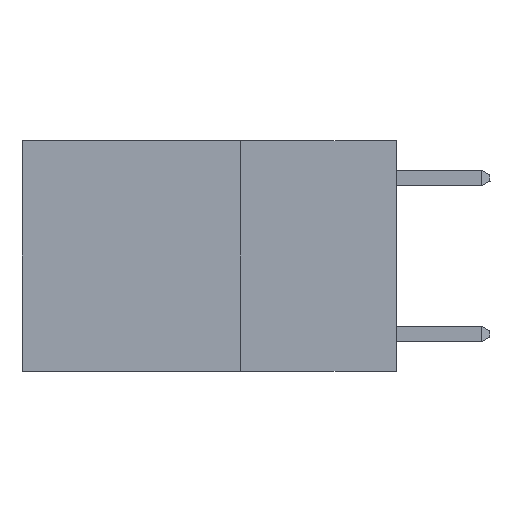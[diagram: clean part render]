
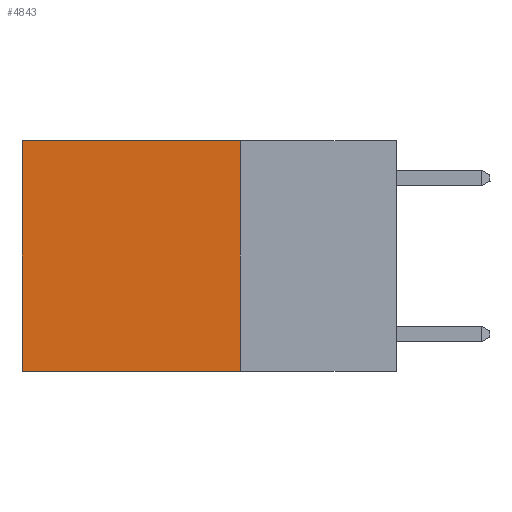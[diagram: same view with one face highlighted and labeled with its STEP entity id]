
A CAD part, left-side view. The second image highlights one B-rep face of the part: STEP entity #4843.
In plain terms, the highlighted planar face has unit normal (-1, 0, 0).
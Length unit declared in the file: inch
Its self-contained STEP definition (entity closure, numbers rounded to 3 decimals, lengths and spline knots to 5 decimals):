
#324 = EDGE_LOOP ( 'NONE', ( #731, #6170, #7046, #10749 ) ) ;
#694 = CARTESIAN_POINT ( 'NONE',  ( 0.2625, 0.25, 0. ) ) ;
#731 = ORIENTED_EDGE ( 'NONE', *, *, #8200, .T. ) ;
#761 = CARTESIAN_POINT ( 'NONE',  ( 0.2625, 0.25, 0. ) ) ;
#950 = DIRECTION ( 'NONE',  ( 0., 1., 0. ) ) ;
#1042 = LINE ( 'NONE', #694, #6366 ) ;
#1320 = DIRECTION ( 'NONE',  ( 0., 0., -1. ) ) ;
#1477 = CARTESIAN_POINT ( 'NONE',  ( 0.2625, 0.6, 0. ) ) ;
#1602 = CARTESIAN_POINT ( 'NONE',  ( 0.2625, 0.25, 0. ) ) ;
#2313 = DIRECTION ( 'NONE',  ( 0., 0., -1. ) ) ;
#2990 = AXIS2_PLACEMENT_3D ( 'NONE', #761, #7392, #2313 ) ;
#3279 = CARTESIAN_POINT ( 'NONE',  ( 0.2625, 0.25, -0.37 ) ) ;
#3387 = LINE ( 'NONE', #4454, #7149 ) ;
#3473 = LINE ( 'NONE', #10647, #9491 ) ;
#3931 = EDGE_CURVE ( 'NONE', #10373, #10743, #11001, .T. ) ;
#4454 = CARTESIAN_POINT ( 'NONE',  ( 0.2625, 0.25, 0. ) ) ;
#4843 = ADVANCED_FACE ( 'NONE', ( #4949 ), #4900, .F. ) ;
#4900 = PLANE ( 'NONE',  #2990 ) ;
#4949 = FACE_OUTER_BOUND ( 'NONE', #324, .T. ) ;
#6170 = ORIENTED_EDGE ( 'NONE', *, *, #3931, .F. ) ;
#6366 = VECTOR ( 'NONE', #10824, 39.37008 ) ;
#6766 = EDGE_CURVE ( 'NONE', #7752, #9865, #3387, .T. ) ;
#7046 = ORIENTED_EDGE ( 'NONE', *, *, #7432, .F. ) ;
#7149 = VECTOR ( 'NONE', #10443, 39.37008 ) ;
#7392 = DIRECTION ( 'NONE',  ( 1., 0., 0. ) ) ;
#7432 = EDGE_CURVE ( 'NONE', #7752, #10373, #1042, .T. ) ;
#7488 = CARTESIAN_POINT ( 'NONE',  ( 0.2625, 0.6, -0.37 ) ) ;
#7752 = VERTEX_POINT ( 'NONE', #1602 ) ;
#8200 = EDGE_CURVE ( 'NONE', #9865, #10743, #3473, .T. ) ;
#9491 = VECTOR ( 'NONE', #1320, 39.37008 ) ;
#9865 = VERTEX_POINT ( 'NONE', #1477 ) ;
#10373 = VERTEX_POINT ( 'NONE', #10933 ) ;
#10443 = DIRECTION ( 'NONE',  ( 0., 1., 0. ) ) ;
#10647 = CARTESIAN_POINT ( 'NONE',  ( 0.2625, 0.6, 0. ) ) ;
#10731 = VECTOR ( 'NONE', #950, 39.37008 ) ;
#10743 = VERTEX_POINT ( 'NONE', #7488 ) ;
#10749 = ORIENTED_EDGE ( 'NONE', *, *, #6766, .T. ) ;
#10824 = DIRECTION ( 'NONE',  ( 0., 0., -1. ) ) ;
#10933 = CARTESIAN_POINT ( 'NONE',  ( 0.2625, 0.25, -0.37 ) ) ;
#11001 = LINE ( 'NONE', #3279, #10731 ) ;
